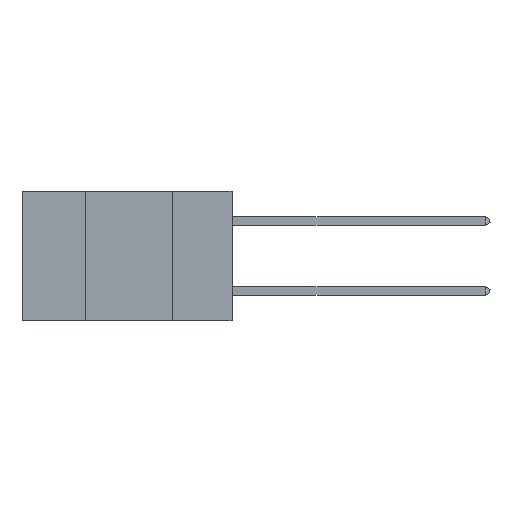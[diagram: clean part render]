
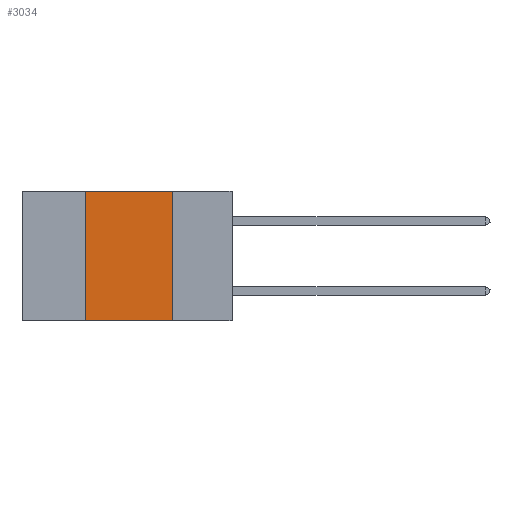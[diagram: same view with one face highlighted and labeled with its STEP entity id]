
A CAD part, left-side view. The second image highlights one B-rep face of the part: STEP entity #3034.
In plain terms, the highlighted planar face has unit normal (-1, 0, 0).
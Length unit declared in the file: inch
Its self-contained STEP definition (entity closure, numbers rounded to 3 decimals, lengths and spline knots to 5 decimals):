
#1092 = CARTESIAN_POINT ( 'NONE',  ( 0., 0.17, 0. ) ) ;
#1149 = FACE_OUTER_BOUND ( 'NONE', #11220, .T. ) ;
#2254 = CARTESIAN_POINT ( 'NONE',  ( 0., 0.6, 0. ) ) ;
#3034 = ADVANCED_FACE ( 'NONE', ( #1149 ), #5077, .F. ) ;
#3290 = CARTESIAN_POINT ( 'NONE',  ( 0., 0.42, -0.37 ) ) ;
#4337 = VERTEX_POINT ( 'NONE', #16822 ) ;
#4976 = CARTESIAN_POINT ( 'NONE',  ( 0., 0.6, -0.37 ) ) ;
#5077 = PLANE ( 'NONE',  #15555 ) ;
#5468 = VERTEX_POINT ( 'NONE', #5496 ) ;
#5496 = CARTESIAN_POINT ( 'NONE',  ( 0., 0.17, 0. ) ) ;
#7990 = EDGE_CURVE ( 'NONE', #5468, #4337, #11113, .T. ) ;
#8106 = VERTEX_POINT ( 'NONE', #13475 ) ;
#8569 = CARTESIAN_POINT ( 'NONE',  ( 0., 0.42, 0. ) ) ;
#9022 = DIRECTION ( 'NONE',  ( 0., -1., 0. ) ) ;
#9123 = DIRECTION ( 'NONE',  ( 0., 0., -1. ) ) ;
#9597 = LINE ( 'NONE', #8569, #10026 ) ;
#9911 = DIRECTION ( 'NONE',  ( 0., 0., 1. ) ) ;
#9924 = ORIENTED_EDGE ( 'NONE', *, *, #13617, .F. ) ;
#10017 = CARTESIAN_POINT ( 'NONE',  ( 0., 0.6, 0. ) ) ;
#10026 = VECTOR ( 'NONE', #9911, 39.37008 ) ;
#10351 = ORIENTED_EDGE ( 'NONE', *, *, #16798, .F. ) ;
#10671 = DIRECTION ( 'NONE',  ( 0., 0., -1. ) ) ;
#11113 = LINE ( 'NONE', #1092, #11509 ) ;
#11127 = VERTEX_POINT ( 'NONE', #3290 ) ;
#11220 = EDGE_LOOP ( 'NONE', ( #14047, #9924, #10351, #12859 ) ) ;
#11390 = LINE ( 'NONE', #10017, #14466 ) ;
#11509 = VECTOR ( 'NONE', #10671, 39.37008 ) ;
#11906 = EDGE_CURVE ( 'NONE', #11127, #4337, #15666, .T. ) ;
#12859 = ORIENTED_EDGE ( 'NONE', *, *, #11906, .T. ) ;
#13475 = CARTESIAN_POINT ( 'NONE',  ( 0., 0.42, 0. ) ) ;
#13617 = EDGE_CURVE ( 'NONE', #8106, #5468, #11390, .T. ) ;
#14047 = ORIENTED_EDGE ( 'NONE', *, *, #7990, .F. ) ;
#14466 = VECTOR ( 'NONE', #16544, 39.37008 ) ;
#15260 = VECTOR ( 'NONE', #9022, 39.37008 ) ;
#15555 = AXIS2_PLACEMENT_3D ( 'NONE', #2254, #16967, #9123 ) ;
#15666 = LINE ( 'NONE', #4976, #15260 ) ;
#16544 = DIRECTION ( 'NONE',  ( 0., -1., 0. ) ) ;
#16798 = EDGE_CURVE ( 'NONE', #11127, #8106, #9597, .T. ) ;
#16822 = CARTESIAN_POINT ( 'NONE',  ( 0., 0.17, -0.37 ) ) ;
#16967 = DIRECTION ( 'NONE',  ( 1., 0., 0. ) ) ;
